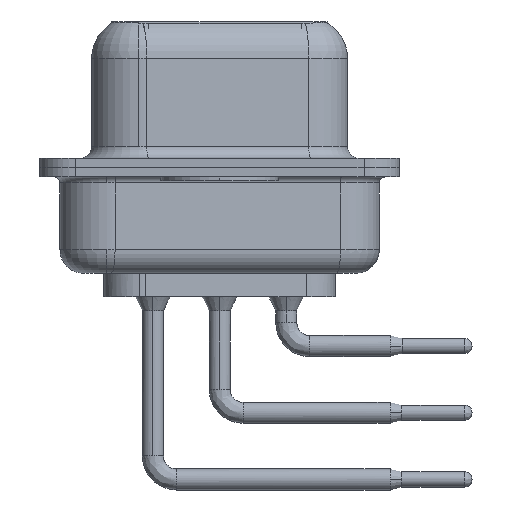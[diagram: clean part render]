
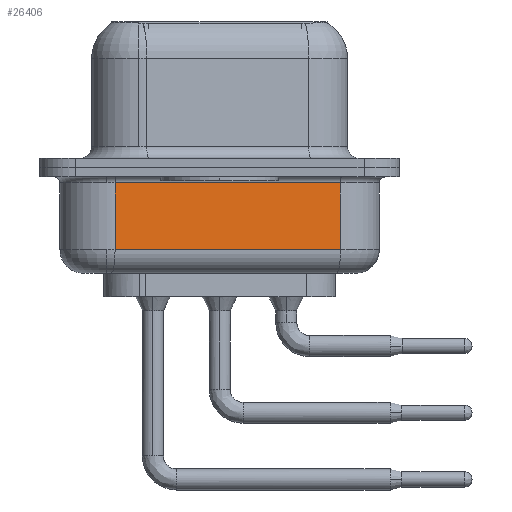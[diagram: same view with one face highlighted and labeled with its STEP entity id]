
A CAD part, left-side view. The second image highlights one B-rep face of the part: STEP entity #26406.
In plain terms, the highlighted planar face has unit normal (-0.985, -0.174, 0).
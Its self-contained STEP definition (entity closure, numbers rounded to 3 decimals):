
#1104 = DIRECTION ( 'NONE',  ( 0.985, 0.174, 0. ) ) ;
#1490 = FACE_OUTER_BOUND ( 'NONE', #24112, .T. ) ;
#1840 = VERTEX_POINT ( 'NONE', #26753 ) ;
#2610 = ORIENTED_EDGE ( 'NONE', *, *, #16786, .T. ) ;
#2787 = EDGE_CURVE ( 'NONE', #16796, #27666, #15451, .T. ) ;
#4213 = AXIS2_PLACEMENT_3D ( 'NONE', #8425, #1104, #18022 ) ;
#4798 = LINE ( 'NONE', #14396, #23899 ) ;
#6938 = EDGE_CURVE ( 'NONE', #27666, #1840, #4798, .T. ) ;
#7279 = CARTESIAN_POINT ( 'NONE',  ( 2.93, 4.453, -0.65 ) ) ;
#8425 = CARTESIAN_POINT ( 'NONE',  ( 2.93, 4.453, -4.5 ) ) ;
#8593 = CARTESIAN_POINT ( 'NONE',  ( 2.93, 4.453, -4.5 ) ) ;
#11896 = EDGE_CURVE ( 'NONE', #16796, #16027, #25559, .T. ) ;
#12223 = LINE ( 'NONE', #12660, #30719 ) ;
#12660 = CARTESIAN_POINT ( 'NONE',  ( 2.93, 4.453, -0.65 ) ) ;
#13972 = DIRECTION ( 'NONE',  ( 0., 0., 1. ) ) ;
#14396 = CARTESIAN_POINT ( 'NONE',  ( 4.623, -5.147, -4.5 ) ) ;
#14521 = ORIENTED_EDGE ( 'NONE', *, *, #2787, .T. ) ;
#15451 = LINE ( 'NONE', #25326, #21069 ) ;
#15643 = CARTESIAN_POINT ( 'NONE',  ( 4.623, -5.147, -3.5 ) ) ;
#16027 = VERTEX_POINT ( 'NONE', #7279 ) ;
#16786 = EDGE_CURVE ( 'NONE', #1840, #16027, #12223, .T. ) ;
#16796 = VERTEX_POINT ( 'NONE', #22274 ) ;
#17135 = ORIENTED_EDGE ( 'NONE', *, *, #11896, .F. ) ;
#18022 = DIRECTION ( 'NONE',  ( -0.174, 0.985, 0. ) ) ;
#18415 = ORIENTED_EDGE ( 'NONE', *, *, #6938, .T. ) ;
#19958 = VECTOR ( 'NONE', #25310, 1000. ) ;
#21069 = VECTOR ( 'NONE', #25174, 1000. ) ;
#22274 = CARTESIAN_POINT ( 'NONE',  ( 2.93, 4.453, -3.5 ) ) ;
#22735 = PLANE ( 'NONE',  #4213 ) ;
#23899 = VECTOR ( 'NONE', #13972, 1000. ) ;
#24112 = EDGE_LOOP ( 'NONE', ( #17135, #14521, #18415, #2610 ) ) ;
#24570 = DIRECTION ( 'NONE',  ( -0.174, 0.985, 0. ) ) ;
#25174 = DIRECTION ( 'NONE',  ( 0.174, -0.985, 0. ) ) ;
#25310 = DIRECTION ( 'NONE',  ( 0., 0., 1. ) ) ;
#25326 = CARTESIAN_POINT ( 'NONE',  ( 2.93, 4.453, -3.5 ) ) ;
#25559 = LINE ( 'NONE', #8593, #19958 ) ;
#26406 = ADVANCED_FACE ( 'NONE', ( #1490 ), #22735, .F. ) ;
#26753 = CARTESIAN_POINT ( 'NONE',  ( 4.623, -5.147, -0.65 ) ) ;
#27666 = VERTEX_POINT ( 'NONE', #15643 ) ;
#30719 = VECTOR ( 'NONE', #24570, 1000. ) ;
